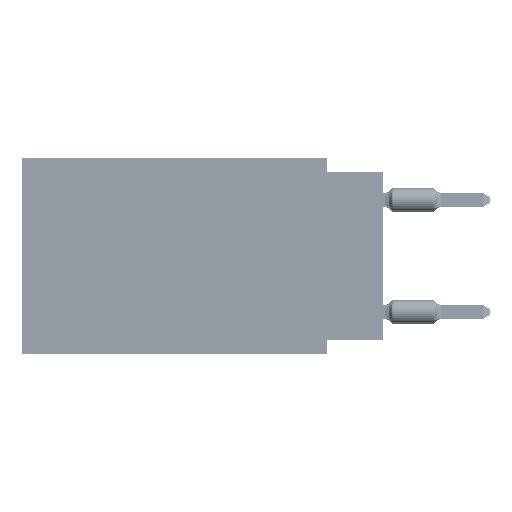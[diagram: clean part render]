
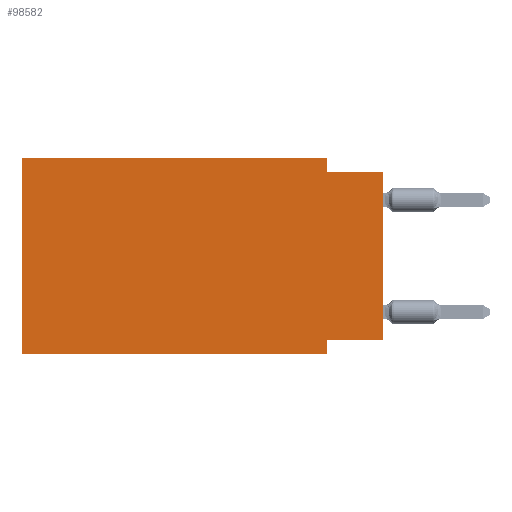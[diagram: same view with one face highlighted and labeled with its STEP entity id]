
A CAD part, left-side view. The second image highlights one B-rep face of the part: STEP entity #98582.
In plain terms, the highlighted planar face has unit normal (-1, 0, 0).
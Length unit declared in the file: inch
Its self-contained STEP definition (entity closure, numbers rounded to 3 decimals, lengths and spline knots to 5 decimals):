
#304 = FACE_OUTER_BOUND ( 'NONE', #31824, .T. ) ;
#491 = CARTESIAN_POINT ( 'NONE',  ( 0., 0.1, -0.025 ) ) ;
#1110 = EDGE_CURVE ( 'NONE', #20363, #97982, #90365, .T. ) ;
#1843 = DIRECTION ( 'NONE',  ( 1., 0., 0. ) ) ;
#2357 = VERTEX_POINT ( 'NONE', #22367 ) ;
#4529 = LINE ( 'NONE', #18647, #93564 ) ;
#7848 = CARTESIAN_POINT ( 'NONE',  ( 0., 0., -0.325 ) ) ;
#8361 = VERTEX_POINT ( 'NONE', #14817 ) ;
#10652 = VERTEX_POINT ( 'NONE', #45373 ) ;
#10789 = DIRECTION ( 'NONE',  ( 0., 0., 1. ) ) ;
#14705 = VECTOR ( 'NONE', #74758, 39.37008 ) ;
#14817 = CARTESIAN_POINT ( 'NONE',  ( 0., 0.1, -0.35 ) ) ;
#16761 = CARTESIAN_POINT ( 'NONE',  ( 0., 0.1, 0. ) ) ;
#18615 = CARTESIAN_POINT ( 'NONE',  ( 0., 0., 0. ) ) ;
#18647 = CARTESIAN_POINT ( 'NONE',  ( 0., 0., -0.325 ) ) ;
#20015 = EDGE_CURVE ( 'NONE', #62084, #29910, #102253, .T. ) ;
#20363 = VERTEX_POINT ( 'NONE', #7848 ) ;
#21543 = CARTESIAN_POINT ( 'NONE',  ( 0., 0., -0.025 ) ) ;
#22367 = CARTESIAN_POINT ( 'NONE',  ( 0., 0.645, -0.35 ) ) ;
#23838 = CARTESIAN_POINT ( 'NONE',  ( 0., 0.645, 0. ) ) ;
#26537 = LINE ( 'NONE', #67370, #14705 ) ;
#27714 = EDGE_CURVE ( 'NONE', #51947, #97982, #95097, .T. ) ;
#28330 = VECTOR ( 'NONE', #30451, 39.37008 ) ;
#29910 = VERTEX_POINT ( 'NONE', #93827 ) ;
#30451 = DIRECTION ( 'NONE',  ( 0., -1., 0. ) ) ;
#30660 = DIRECTION ( 'NONE',  ( 0., -1., 0. ) ) ;
#31824 = EDGE_LOOP ( 'NONE', ( #49659, #75486, #71538, #40118, #49264, #63907, #68905, #89857 ) ) ;
#34201 = VECTOR ( 'NONE', #30660, 39.37008 ) ;
#39355 = CARTESIAN_POINT ( 'NONE',  ( 0., 0.645, 0. ) ) ;
#40118 = ORIENTED_EDGE ( 'NONE', *, *, #20015, .F. ) ;
#41059 = VECTOR ( 'NONE', #63673, 39.37008 ) ;
#42740 = DIRECTION ( 'NONE',  ( 0., 1., 0. ) ) ;
#45144 = CARTESIAN_POINT ( 'NONE',  ( 0., 0.645, 0. ) ) ;
#45373 = CARTESIAN_POINT ( 'NONE',  ( 0., 0.1, -0.325 ) ) ;
#45913 = LINE ( 'NONE', #55303, #41059 ) ;
#48945 = PLANE ( 'NONE',  #61689 ) ;
#49264 = ORIENTED_EDGE ( 'NONE', *, *, #57353, .F. ) ;
#49659 = ORIENTED_EDGE ( 'NONE', *, *, #1110, .T. ) ;
#51947 = VERTEX_POINT ( 'NONE', #491 ) ;
#54760 = CARTESIAN_POINT ( 'NONE',  ( 0., 0., -0.025 ) ) ;
#55303 = CARTESIAN_POINT ( 'NONE',  ( 0., 0.1, -0.35 ) ) ;
#57301 = DIRECTION ( 'NONE',  ( 0., 0., -1. ) ) ;
#57353 = EDGE_CURVE ( 'NONE', #2357, #62084, #61868, .T. ) ;
#61193 = EDGE_CURVE ( 'NONE', #10652, #8361, #45913, .T. ) ;
#61689 = AXIS2_PLACEMENT_3D ( 'NONE', #23838, #1843, #57301 ) ;
#61868 = LINE ( 'NONE', #45144, #83482 ) ;
#62084 = VERTEX_POINT ( 'NONE', #65350 ) ;
#63673 = DIRECTION ( 'NONE',  ( 0., 0., -1. ) ) ;
#63907 = ORIENTED_EDGE ( 'NONE', *, *, #86392, .T. ) ;
#65350 = CARTESIAN_POINT ( 'NONE',  ( 0., 0.645, 0. ) ) ;
#67370 = CARTESIAN_POINT ( 'NONE',  ( 0., 0.645, -0.35 ) ) ;
#68905 = ORIENTED_EDGE ( 'NONE', *, *, #61193, .F. ) ;
#69023 = EDGE_CURVE ( 'NONE', #20363, #10652, #4529, .T. ) ;
#69291 = VECTOR ( 'NONE', #10789, 39.37008 ) ;
#71538 = ORIENTED_EDGE ( 'NONE', *, *, #88925, .F. ) ;
#74758 = DIRECTION ( 'NONE',  ( 0., -1., 0. ) ) ;
#75486 = ORIENTED_EDGE ( 'NONE', *, *, #27714, .F. ) ;
#77529 = VECTOR ( 'NONE', #94831, 39.37008 ) ;
#83482 = VECTOR ( 'NONE', #84960, 39.37008 ) ;
#84960 = DIRECTION ( 'NONE',  ( 0., 0., 1. ) ) ;
#86392 = EDGE_CURVE ( 'NONE', #2357, #8361, #26537, .T. ) ;
#88925 = EDGE_CURVE ( 'NONE', #29910, #51947, #96380, .T. ) ;
#89857 = ORIENTED_EDGE ( 'NONE', *, *, #69023, .F. ) ;
#90365 = LINE ( 'NONE', #18615, #69291 ) ;
#93564 = VECTOR ( 'NONE', #42740, 39.37008 ) ;
#93827 = CARTESIAN_POINT ( 'NONE',  ( 0., 0.1, 0. ) ) ;
#94831 = DIRECTION ( 'NONE',  ( 0., 0., -1. ) ) ;
#95097 = LINE ( 'NONE', #54760, #34201 ) ;
#96380 = LINE ( 'NONE', #16761, #77529 ) ;
#97982 = VERTEX_POINT ( 'NONE', #21543 ) ;
#98582 = ADVANCED_FACE ( 'NONE', ( #304 ), #48945, .F. ) ;
#102253 = LINE ( 'NONE', #39355, #28330 ) ;
